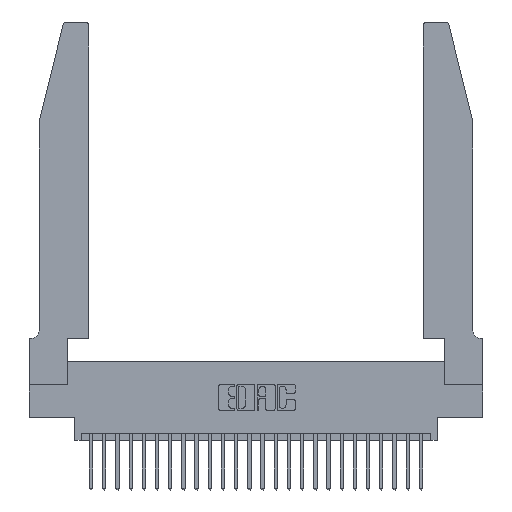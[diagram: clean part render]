
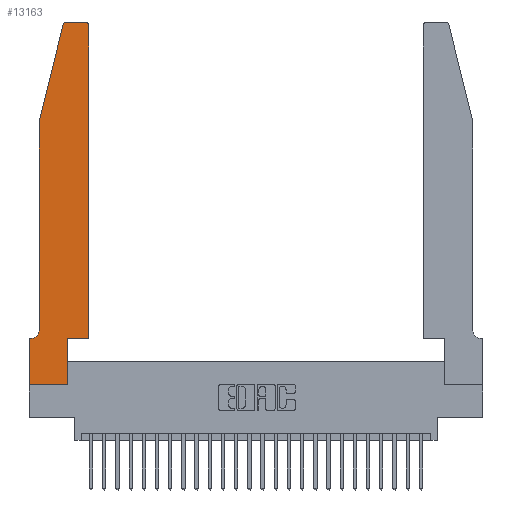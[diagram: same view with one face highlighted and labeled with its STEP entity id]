
A CAD part, top view. The second image highlights one B-rep face of the part: STEP entity #13163.
In plain terms, the highlighted planar face has unit normal (0, 0, 1).
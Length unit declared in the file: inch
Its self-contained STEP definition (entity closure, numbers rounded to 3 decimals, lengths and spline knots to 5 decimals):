
#302 = LINE ( 'NONE', #8215, #11086 ) ;
#2218 = CARTESIAN_POINT ( 'NONE',  ( 0.0755, 0.42, 0.37 ) ) ;
#2260 = EDGE_CURVE ( 'NONE', #22664, #10078, #17767, .T. ) ;
#2355 = EDGE_CURVE ( 'NONE', #26687, #16059, #21368, .T. ) ;
#2406 = EDGE_CURVE ( 'NONE', #3310, #3133, #19397, .T. ) ;
#2495 = LINE ( 'NONE', #10657, #18851 ) ;
#2556 = AXIS2_PLACEMENT_3D ( 'NONE', #20046, #7387, #22165 ) ;
#3133 = VERTEX_POINT ( 'NONE', #17349 ) ;
#3310 = VERTEX_POINT ( 'NONE', #13598 ) ;
#3342 = ORIENTED_EDGE ( 'NONE', *, *, #22216, .T. ) ;
#3762 = LINE ( 'NONE', #26146, #20033 ) ;
#3997 = DIRECTION ( 'NONE',  ( 0., -1., 0. ) ) ;
#4150 = ORIENTED_EDGE ( 'NONE', *, *, #2406, .T. ) ;
#4722 = VERTEX_POINT ( 'NONE', #14068 ) ;
#4882 = EDGE_CURVE ( 'NONE', #10078, #16779, #302, .T. ) ;
#5691 = ORIENTED_EDGE ( 'NONE', *, *, #19334, .T. ) ;
#6277 = LINE ( 'NONE', #13731, #16897 ) ;
#6327 = DIRECTION ( 'NONE',  ( 0., -1., 0. ) ) ;
#6593 = VECTOR ( 'NONE', #6327, 39.37008 ) ;
#6775 = DIRECTION ( 'NONE',  ( 1., 0., 0. ) ) ;
#7387 = DIRECTION ( 'NONE',  ( 0., 0., 1. ) ) ;
#7495 = DIRECTION ( 'NONE',  ( 0., 0., -1. ) ) ;
#7905 = LINE ( 'NONE', #19188, #11573 ) ;
#7980 = CARTESIAN_POINT ( 'NONE',  ( 0.4505, 0.35, 0.37 ) ) ;
#8042 = EDGE_CURVE ( 'NONE', #16059, #19412, #8965, .T. ) ;
#8215 = CARTESIAN_POINT ( 'NONE',  ( 0.0755, 0.35, 0.37 ) ) ;
#8965 = CIRCLE ( 'NONE', #10133, 0.03 ) ;
#9028 = ORIENTED_EDGE ( 'NONE', *, *, #19037, .T. ) ;
#9630 = LINE ( 'NONE', #18865, #20155 ) ;
#10024 = CARTESIAN_POINT ( 'NONE',  ( 0.2605, 2.75, 0.37 ) ) ;
#10078 = VERTEX_POINT ( 'NONE', #14842 ) ;
#10133 = AXIS2_PLACEMENT_3D ( 'NONE', #24903, #12335, #27025 ) ;
#10650 = CARTESIAN_POINT ( 'NONE',  ( 0.25487, 2.72718, 0.37 ) ) ;
#10657 = CARTESIAN_POINT ( 'NONE',  ( 0.2865, 0.35, 0.37 ) ) ;
#10804 = DIRECTION ( 'NONE',  ( 1., 0., 0. ) ) ;
#11086 = VECTOR ( 'NONE', #27169, 39.37008 ) ;
#11101 = ORIENTED_EDGE ( 'NONE', *, *, #8042, .T. ) ;
#11469 = DIRECTION ( 'NONE',  ( 1., 0., 0. ) ) ;
#11573 = VECTOR ( 'NONE', #10804, 39.37008 ) ;
#11694 = ORIENTED_EDGE ( 'NONE', *, *, #2355, .T. ) ;
#12167 = DIRECTION ( 'NONE',  ( -1., 0., 0. ) ) ;
#12335 = DIRECTION ( 'NONE',  ( 0., 0., 1. ) ) ;
#13163 = ADVANCED_FACE ( 'NONE', ( #15636 ), #20619, .T. ) ;
#13598 = CARTESIAN_POINT ( 'NONE',  ( 0.4505, 0.35, 0.37 ) ) ;
#13731 = CARTESIAN_POINT ( 'NONE',  ( 0.0755, 2., 0.37 ) ) ;
#13828 = VECTOR ( 'NONE', #18598, 39.37008 ) ;
#14068 = CARTESIAN_POINT ( 'NONE',  ( 0., 0., 0.37 ) ) ;
#14482 = EDGE_CURVE ( 'NONE', #15031, #18024, #2495, .T. ) ;
#14842 = CARTESIAN_POINT ( 'NONE',  ( 0.0055, 0.35, 0.37 ) ) ;
#14987 = EDGE_CURVE ( 'NONE', #16145, #22664, #18542, .T. ) ;
#15031 = VERTEX_POINT ( 'NONE', #21208 ) ;
#15153 = VECTOR ( 'NONE', #12167, 39.37008 ) ;
#15256 = CARTESIAN_POINT ( 'NONE',  ( 0., 0.35, 0.37 ) ) ;
#15636 = FACE_OUTER_BOUND ( 'NONE', #22471, .T. ) ;
#15852 = DIRECTION ( 'NONE',  ( -0.239, -0.971, 0. ) ) ;
#16059 = VERTEX_POINT ( 'NONE', #20618 ) ;
#16145 = VERTEX_POINT ( 'NONE', #19593 ) ;
#16779 = VERTEX_POINT ( 'NONE', #26450 ) ;
#16897 = VECTOR ( 'NONE', #15852, 39.37008 ) ;
#17349 = CARTESIAN_POINT ( 'NONE',  ( 0.4505, 2.72, 0.37 ) ) ;
#17495 = ORIENTED_EDGE ( 'NONE', *, *, #4882, .T. ) ;
#17767 = CIRCLE ( 'NONE', #25652, 0.07 ) ;
#17795 = AXIS2_PLACEMENT_3D ( 'NONE', #15256, #19460, #6775 ) ;
#18024 = VERTEX_POINT ( 'NONE', #20331 ) ;
#18542 = LINE ( 'NONE', #25240, #6593 ) ;
#18598 = DIRECTION ( 'NONE',  ( 0., 1., 0. ) ) ;
#18821 = ORIENTED_EDGE ( 'NONE', *, *, #2260, .T. ) ;
#18851 = VECTOR ( 'NONE', #27468, 39.37008 ) ;
#18865 = CARTESIAN_POINT ( 'NONE',  ( 0., 0., 0.37 ) ) ;
#19037 = EDGE_CURVE ( 'NONE', #19412, #16145, #6277, .T. ) ;
#19188 = CARTESIAN_POINT ( 'NONE',  ( 0.4505, 0.35, 0.37 ) ) ;
#19334 = EDGE_CURVE ( 'NONE', #16779, #4722, #9630, .T. ) ;
#19397 = LINE ( 'NONE', #7980, #13828 ) ;
#19412 = VERTEX_POINT ( 'NONE', #10650 ) ;
#19460 = DIRECTION ( 'NONE',  ( 0., 0., 1. ) ) ;
#19593 = CARTESIAN_POINT ( 'NONE',  ( 0.0755, 2., 0.37 ) ) ;
#20033 = VECTOR ( 'NONE', #11469, 39.37008 ) ;
#20046 = CARTESIAN_POINT ( 'NONE',  ( 0.4205, 2.72, 0.37 ) ) ;
#20132 = EDGE_CURVE ( 'NONE', #18024, #3310, #7905, .T. ) ;
#20150 = CARTESIAN_POINT ( 'NONE',  ( 0.0055, 0.42, 0.37 ) ) ;
#20155 = VECTOR ( 'NONE', #3997, 39.37008 ) ;
#20331 = CARTESIAN_POINT ( 'NONE',  ( 0.2865, 0.35, 0.37 ) ) ;
#20619 = PLANE ( 'NONE',  #17795 ) ;
#20618 = CARTESIAN_POINT ( 'NONE',  ( 0.284, 2.75, 0.37 ) ) ;
#21006 = EDGE_CURVE ( 'NONE', #3133, #26687, #25037, .T. ) ;
#21208 = CARTESIAN_POINT ( 'NONE',  ( 0.2865, 0., 0.37 ) ) ;
#21368 = LINE ( 'NONE', #10024, #15153 ) ;
#22042 = ORIENTED_EDGE ( 'NONE', *, *, #20132, .T. ) ;
#22165 = DIRECTION ( 'NONE',  ( 1., 0., 0. ) ) ;
#22216 = EDGE_CURVE ( 'NONE', #4722, #15031, #3762, .T. ) ;
#22268 = DIRECTION ( 'NONE',  ( -1., 0., 0. ) ) ;
#22471 = EDGE_LOOP ( 'NONE', ( #11694, #11101, #9028, #23303, #18821, #17495, #5691, #3342, #24202, #22042, #4150, #23502 ) ) ;
#22664 = VERTEX_POINT ( 'NONE', #2218 ) ;
#22793 = CARTESIAN_POINT ( 'NONE',  ( 0.4205, 2.75, 0.37 ) ) ;
#23303 = ORIENTED_EDGE ( 'NONE', *, *, #14987, .T. ) ;
#23502 = ORIENTED_EDGE ( 'NONE', *, *, #21006, .T. ) ;
#24202 = ORIENTED_EDGE ( 'NONE', *, *, #14482, .T. ) ;
#24903 = CARTESIAN_POINT ( 'NONE',  ( 0.284, 2.72, 0.37 ) ) ;
#25037 = CIRCLE ( 'NONE', #2556, 0.03 ) ;
#25240 = CARTESIAN_POINT ( 'NONE',  ( 0.0755, 2., 0.37 ) ) ;
#25652 = AXIS2_PLACEMENT_3D ( 'NONE', #20150, #7495, #22268 ) ;
#26146 = CARTESIAN_POINT ( 'NONE',  ( 0., 0., 0.37 ) ) ;
#26450 = CARTESIAN_POINT ( 'NONE',  ( 0., 0.35, 0.37 ) ) ;
#26687 = VERTEX_POINT ( 'NONE', #22793 ) ;
#27025 = DIRECTION ( 'NONE',  ( 1., 0., 0. ) ) ;
#27169 = DIRECTION ( 'NONE',  ( -1., 0., 0. ) ) ;
#27468 = DIRECTION ( 'NONE',  ( 0., 1., 0. ) ) ;
